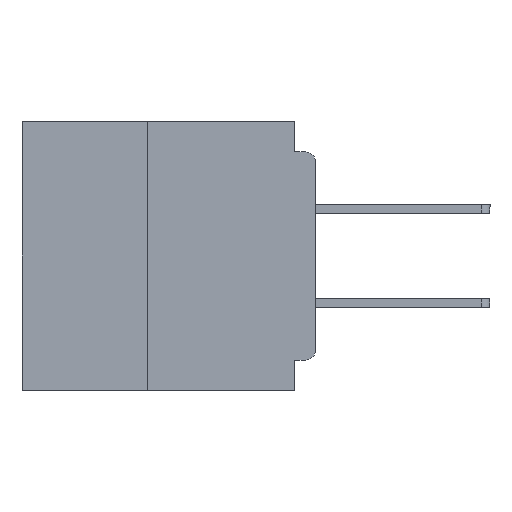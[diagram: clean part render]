
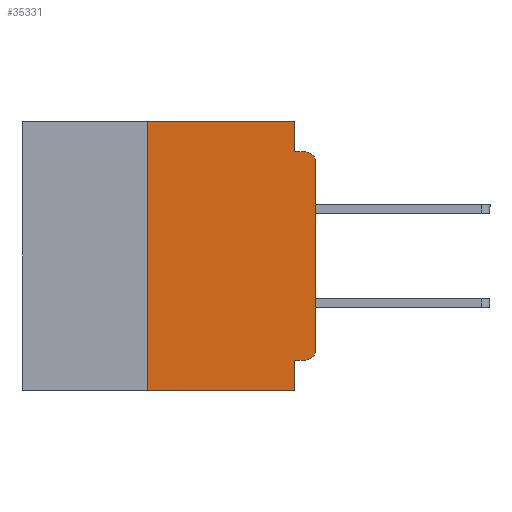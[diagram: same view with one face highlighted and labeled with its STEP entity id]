
A CAD part, left-side view. The second image highlights one B-rep face of the part: STEP entity #35331.
In plain terms, the highlighted planar face has unit normal (-1, 0, 0).
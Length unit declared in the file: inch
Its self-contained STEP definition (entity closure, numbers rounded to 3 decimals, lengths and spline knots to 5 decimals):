
#1131 = EDGE_CURVE ( 'NONE', #2588, #4618, #1673, .T. ) ;
#1673 = LINE ( 'NONE', #38792, #27763 ) ;
#2201 = CARTESIAN_POINT ( 'NONE',  ( 0., 0., -0.355 ) ) ;
#2254 = CARTESIAN_POINT ( 'NONE',  ( 0., 0.25, 0. ) ) ;
#2456 = CARTESIAN_POINT ( 'NONE',  ( 0., 0.015, -0.06 ) ) ;
#2588 = VERTEX_POINT ( 'NONE', #39869 ) ;
#3210 = VERTEX_POINT ( 'NONE', #47425 ) ;
#3387 = VECTOR ( 'NONE', #47706, 39.37008 ) ;
#4396 = DIRECTION ( 'NONE',  ( 1., 0., 0. ) ) ;
#4618 = VERTEX_POINT ( 'NONE', #44054 ) ;
#5659 = VERTEX_POINT ( 'NONE', #32428 ) ;
#6189 = DIRECTION ( 'NONE',  ( 0., 0., -1. ) ) ;
#6803 = EDGE_CURVE ( 'NONE', #43866, #2588, #29873, .T. ) ;
#7734 = CARTESIAN_POINT ( 'NONE',  ( 0., 0., -0.06 ) ) ;
#8346 = AXIS2_PLACEMENT_3D ( 'NONE', #15152, #40871, #18870 ) ;
#8384 = VERTEX_POINT ( 'NONE', #16005 ) ;
#9034 = VECTOR ( 'NONE', #46257, 39.37008 ) ;
#10829 = ORIENTED_EDGE ( 'NONE', *, *, #31670, .F. ) ;
#11898 = LINE ( 'NONE', #40264, #40094 ) ;
#12474 = CARTESIAN_POINT ( 'NONE',  ( 0., 0., -0.34 ) ) ;
#13203 = ORIENTED_EDGE ( 'NONE', *, *, #21007, .F. ) ;
#13587 = VERTEX_POINT ( 'NONE', #12474 ) ;
#14516 = DIRECTION ( 'NONE',  ( 0., -1., 0. ) ) ;
#15152 = CARTESIAN_POINT ( 'NONE',  ( 0., 0.015, -0.34 ) ) ;
#15348 = CARTESIAN_POINT ( 'NONE',  ( 0., 0.437, 0. ) ) ;
#15558 = VECTOR ( 'NONE', #27387, 39.37008 ) ;
#15827 = EDGE_CURVE ( 'NONE', #13587, #33756, #42547, .T. ) ;
#16005 = CARTESIAN_POINT ( 'NONE',  ( 0., 0.25, -0.4 ) ) ;
#16032 = EDGE_CURVE ( 'NONE', #8384, #4618, #41962, .T. ) ;
#17173 = ORIENTED_EDGE ( 'NONE', *, *, #1131, .F. ) ;
#17664 = EDGE_CURVE ( 'NONE', #43866, #13587, #33014, .T. ) ;
#18522 = EDGE_CURVE ( 'NONE', #8384, #39067, #34061, .T. ) ;
#18870 = DIRECTION ( 'NONE',  ( 0., 0., -1. ) ) ;
#21007 = EDGE_CURVE ( 'NONE', #3210, #5659, #30465, .T. ) ;
#21673 = ORIENTED_EDGE ( 'NONE', *, *, #6803, .F. ) ;
#22228 = VECTOR ( 'NONE', #26518, 39.37008 ) ;
#23959 = CARTESIAN_POINT ( 'NONE',  ( 0., 0.015, -0.045 ) ) ;
#25572 = CARTESIAN_POINT ( 'NONE',  ( 0., 0.031, 0. ) ) ;
#25873 = CARTESIAN_POINT ( 'NONE',  ( 0., 0., 0. ) ) ;
#26518 = DIRECTION ( 'NONE',  ( 0., -1., 0. ) ) ;
#26578 = CARTESIAN_POINT ( 'NONE',  ( 0., 0.437, 0. ) ) ;
#27143 = CARTESIAN_POINT ( 'NONE',  ( 0., 0.437, -0.4 ) ) ;
#27387 = DIRECTION ( 'NONE',  ( 0., 0., 1. ) ) ;
#27763 = VECTOR ( 'NONE', #36748, 39.37008 ) ;
#28309 = EDGE_CURVE ( 'NONE', #39067, #3210, #32104, .T. ) ;
#28390 = DIRECTION ( 'NONE',  ( -1., 0., 0. ) ) ;
#28982 = CARTESIAN_POINT ( 'NONE',  ( 0., 0.015, -0.355 ) ) ;
#29130 = DIRECTION ( 'NONE',  ( 0., 0., -1. ) ) ;
#29873 = LINE ( 'NONE', #2201, #9034 ) ;
#30251 = ORIENTED_EDGE ( 'NONE', *, *, #16032, .T. ) ;
#30321 = DIRECTION ( 'NONE',  ( 0., 0., -1. ) ) ;
#30465 = LINE ( 'NONE', #25572, #37863 ) ;
#31670 = EDGE_CURVE ( 'NONE', #5659, #41028, #11898, .T. ) ;
#32104 = LINE ( 'NONE', #15348, #22228 ) ;
#32347 = VECTOR ( 'NONE', #34398, 39.37008 ) ;
#32428 = CARTESIAN_POINT ( 'NONE',  ( 0., 0.031, -0.045 ) ) ;
#33014 = CIRCLE ( 'NONE', #8346, 0.015 ) ;
#33484 = ORIENTED_EDGE ( 'NONE', *, *, #34997, .T. ) ;
#33756 = VERTEX_POINT ( 'NONE', #7734 ) ;
#34061 = LINE ( 'NONE', #42045, #15558 ) ;
#34398 = DIRECTION ( 'NONE',  ( 0., -1., 0. ) ) ;
#34651 = ORIENTED_EDGE ( 'NONE', *, *, #28309, .F. ) ;
#34918 = ORIENTED_EDGE ( 'NONE', *, *, #18522, .F. ) ;
#34997 = EDGE_CURVE ( 'NONE', #33756, #41028, #44259, .T. ) ;
#35331 = ADVANCED_FACE ( 'NONE', ( #47135 ), #40970, .F. ) ;
#36748 = DIRECTION ( 'NONE',  ( 0., 0., -1. ) ) ;
#37863 = VECTOR ( 'NONE', #29130, 39.37008 ) ;
#38792 = CARTESIAN_POINT ( 'NONE',  ( 0., 0.031, -0.4 ) ) ;
#39067 = VERTEX_POINT ( 'NONE', #2254 ) ;
#39234 = ORIENTED_EDGE ( 'NONE', *, *, #17664, .T. ) ;
#39869 = CARTESIAN_POINT ( 'NONE',  ( 0., 0.031, -0.355 ) ) ;
#40094 = VECTOR ( 'NONE', #14516, 39.37008 ) ;
#40264 = CARTESIAN_POINT ( 'NONE',  ( 0., 0., -0.045 ) ) ;
#40753 = EDGE_LOOP ( 'NONE', ( #44518, #33484, #10829, #13203, #34651, #34918, #30251, #17173, #21673, #39234 ) ) ;
#40871 = DIRECTION ( 'NONE',  ( -1., 0., 0. ) ) ;
#40970 = PLANE ( 'NONE',  #45308 ) ;
#41028 = VERTEX_POINT ( 'NONE', #23959 ) ;
#41359 = AXIS2_PLACEMENT_3D ( 'NONE', #2456, #28390, #6189 ) ;
#41962 = LINE ( 'NONE', #27143, #32347 ) ;
#42045 = CARTESIAN_POINT ( 'NONE',  ( 0., 0.25, -0.4 ) ) ;
#42547 = LINE ( 'NONE', #25873, #3387 ) ;
#43866 = VERTEX_POINT ( 'NONE', #28982 ) ;
#44054 = CARTESIAN_POINT ( 'NONE',  ( 0., 0.031, -0.4 ) ) ;
#44259 = CIRCLE ( 'NONE', #41359, 0.015 ) ;
#44518 = ORIENTED_EDGE ( 'NONE', *, *, #15827, .T. ) ;
#45308 = AXIS2_PLACEMENT_3D ( 'NONE', #26578, #4396, #30321 ) ;
#46257 = DIRECTION ( 'NONE',  ( 0., 1., 0. ) ) ;
#47135 = FACE_OUTER_BOUND ( 'NONE', #40753, .T. ) ;
#47425 = CARTESIAN_POINT ( 'NONE',  ( 0., 0.031, 0. ) ) ;
#47706 = DIRECTION ( 'NONE',  ( 0., 0., 1. ) ) ;
